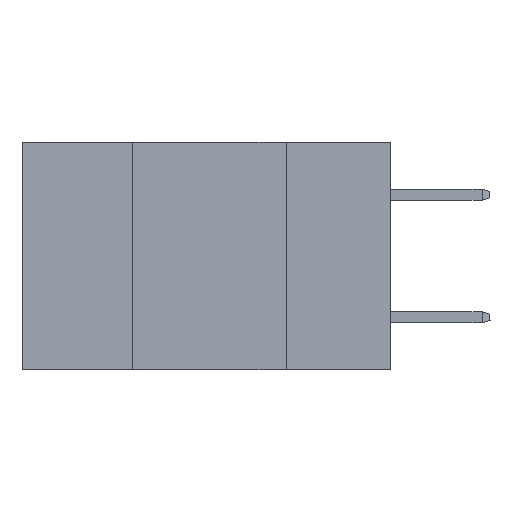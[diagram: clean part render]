
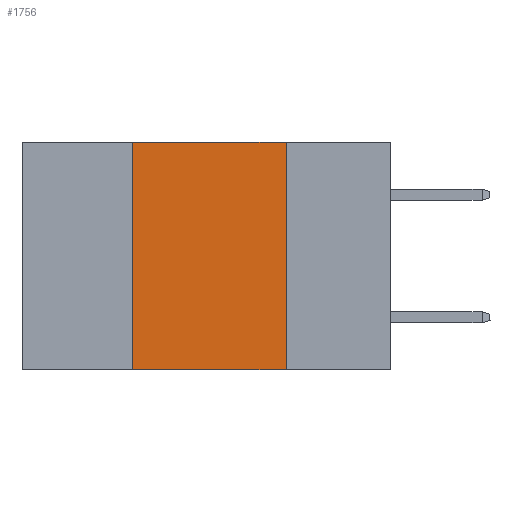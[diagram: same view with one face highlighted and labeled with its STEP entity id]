
A CAD part, left-side view. The second image highlights one B-rep face of the part: STEP entity #1756.
In plain terms, the highlighted planar face has unit normal (-1, 0, 0).
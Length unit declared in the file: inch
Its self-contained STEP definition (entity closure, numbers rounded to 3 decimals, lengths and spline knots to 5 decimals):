
#1756 = ADVANCED_FACE ( 'NONE', ( #23998 ), #5649, .F. ) ;
#3678 = DIRECTION ( 'NONE',  ( 0., 0., 1. ) ) ;
#4296 = VERTEX_POINT ( 'NONE', #19203 ) ;
#4539 = DIRECTION ( 'NONE',  ( 0., -1., 0. ) ) ;
#5649 = PLANE ( 'NONE',  #19553 ) ;
#5798 = ORIENTED_EDGE ( 'NONE', *, *, #23107, .F. ) ;
#6041 = DIRECTION ( 'NONE',  ( 1., 0., 0. ) ) ;
#6919 = LINE ( 'NONE', #17289, #23213 ) ;
#6987 = LINE ( 'NONE', #22265, #8036 ) ;
#7981 = EDGE_CURVE ( 'NONE', #24395, #11606, #19262, .T. ) ;
#8036 = VECTOR ( 'NONE', #4539, 39.37008 ) ;
#8141 = DIRECTION ( 'NONE',  ( 0., -1., 0. ) ) ;
#8840 = EDGE_CURVE ( 'NONE', #11606, #4296, #18878, .T. ) ;
#9187 = ORIENTED_EDGE ( 'NONE', *, *, #8840, .F. ) ;
#9405 = ORIENTED_EDGE ( 'NONE', *, *, #22189, .T. ) ;
#10200 = CARTESIAN_POINT ( 'NONE',  ( 0., 0.6, 0. ) ) ;
#10482 = DIRECTION ( 'NONE',  ( 0., 0., -1. ) ) ;
#10612 = EDGE_LOOP ( 'NONE', ( #9187, #21643, #5798, #9405 ) ) ;
#11606 = VERTEX_POINT ( 'NONE', #21319 ) ;
#13037 = CARTESIAN_POINT ( 'NONE',  ( 0., 0.6, 0. ) ) ;
#13643 = VECTOR ( 'NONE', #8141, 39.37008 ) ;
#17289 = CARTESIAN_POINT ( 'NONE',  ( 0., 0.42, 0. ) ) ;
#17706 = CARTESIAN_POINT ( 'NONE',  ( 0., 0.42, 0. ) ) ;
#18186 = VECTOR ( 'NONE', #19803, 39.37008 ) ;
#18878 = LINE ( 'NONE', #26953, #18186 ) ;
#19203 = CARTESIAN_POINT ( 'NONE',  ( 0., 0.17, -0.37 ) ) ;
#19262 = LINE ( 'NONE', #13037, #13643 ) ;
#19553 = AXIS2_PLACEMENT_3D ( 'NONE', #10200, #6041, #10482 ) ;
#19803 = DIRECTION ( 'NONE',  ( 0., 0., -1. ) ) ;
#21319 = CARTESIAN_POINT ( 'NONE',  ( 0., 0.17, 0. ) ) ;
#21643 = ORIENTED_EDGE ( 'NONE', *, *, #7981, .F. ) ;
#22189 = EDGE_CURVE ( 'NONE', #22374, #4296, #6987, .T. ) ;
#22265 = CARTESIAN_POINT ( 'NONE',  ( 0., 0.6, -0.37 ) ) ;
#22374 = VERTEX_POINT ( 'NONE', #23050 ) ;
#23050 = CARTESIAN_POINT ( 'NONE',  ( 0., 0.42, -0.37 ) ) ;
#23107 = EDGE_CURVE ( 'NONE', #22374, #24395, #6919, .T. ) ;
#23213 = VECTOR ( 'NONE', #3678, 39.37008 ) ;
#23998 = FACE_OUTER_BOUND ( 'NONE', #10612, .T. ) ;
#24395 = VERTEX_POINT ( 'NONE', #17706 ) ;
#26953 = CARTESIAN_POINT ( 'NONE',  ( 0., 0.17, 0. ) ) ;
